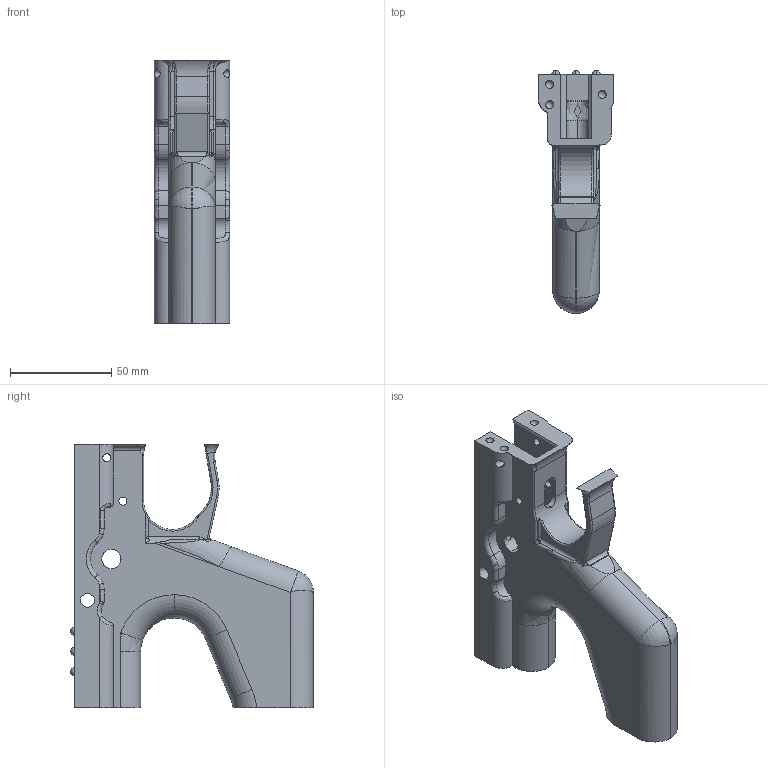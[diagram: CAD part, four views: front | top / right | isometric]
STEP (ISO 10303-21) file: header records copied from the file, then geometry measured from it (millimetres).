
FILE_DESCRIPTION (( 'STEP AP214' ), '1' );
FILE_NAME ('Unbuffered_Pistol_3.STEP', '2015-10-23T19:45:04', ( 'WarFairy' ), ( '' ), 'SwSTEP 2.0', 'SolidWorks 2015', '' );
FILE_SCHEMA (( 'AUTOMOTIVE_DESIGN' ));
Length unit declared in the file: millimetre
Products named in the file (1): Unbuffered_Pistol_3
Bounding box: 37.13 x 119.8 x 130 mm (x, y, z)
Volume: 200277 mm3; surface area: 40387.5 mm2
Topology: 1 solids, 1 shells, 263 faces, 728 edges, 446 vertices
Faces by surface type: cylinder 104, bspline 53, plane 42, torus 39, sphere 25
Entity records: 12200 total; most frequent: CARTESIAN_POINT 6046, ORIENTED_EDGE 1356, DIRECTION 1208, EDGE_CURVE 678, AXIS2_PLACEMENT_3D 494, VERTEX_POINT 427, EDGE_LOOP 293, CIRCLE 283
